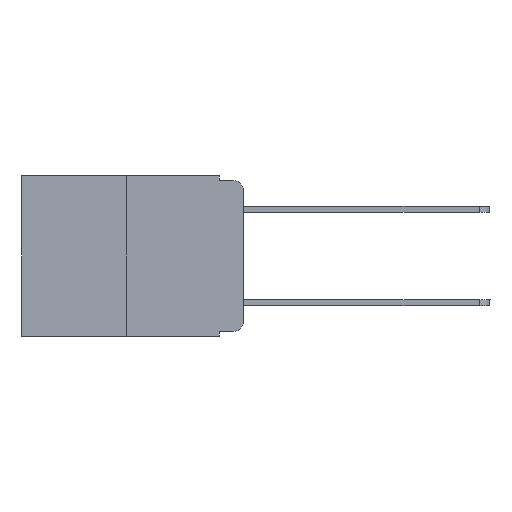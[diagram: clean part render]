
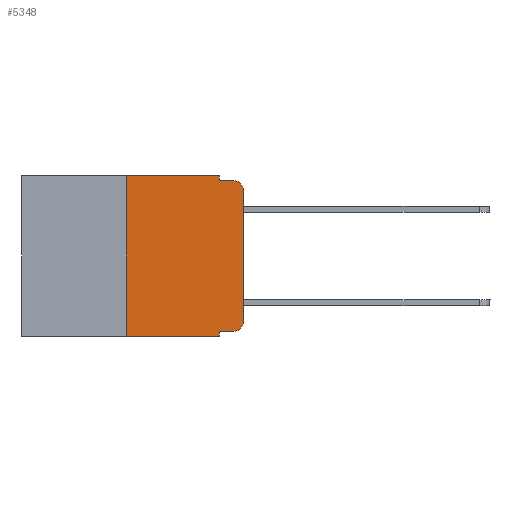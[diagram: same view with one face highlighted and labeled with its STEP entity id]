
A CAD part, left-side view. The second image highlights one B-rep face of the part: STEP entity #5348.
In plain terms, the highlighted planar face has unit normal (-1, 0, 0).
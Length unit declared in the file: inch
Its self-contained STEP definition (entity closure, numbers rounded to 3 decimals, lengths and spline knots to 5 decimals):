
#55 = VERTEX_POINT ( 'NONE', #11391 ) ;
#371 = DIRECTION ( 'NONE',  ( 0., -1., 0. ) ) ;
#463 = CARTESIAN_POINT ( 'NONE',  ( 0., 0.051, -0.01 ) ) ;
#691 = ORIENTED_EDGE ( 'NONE', *, *, #2611, .T. ) ;
#784 = VERTEX_POINT ( 'NONE', #4532 ) ;
#833 = EDGE_CURVE ( 'NONE', #9149, #11149, #3666, .T. ) ;
#1502 = CARTESIAN_POINT ( 'NONE',  ( 0., 0.473, -0.343 ) ) ;
#1610 = PLANE ( 'NONE',  #10020 ) ;
#1618 = CIRCLE ( 'NONE', #2426, 0.02 ) ;
#1732 = CARTESIAN_POINT ( 'NONE',  ( 0., 0., -0.313 ) ) ;
#1734 = DIRECTION ( 'NONE',  ( 0., 0., -1. ) ) ;
#2113 = VERTEX_POINT ( 'NONE', #3865 ) ;
#2253 = CARTESIAN_POINT ( 'NONE',  ( 0., 0.02, -0.333 ) ) ;
#2263 = EDGE_CURVE ( 'NONE', #55, #4100, #9160, .T. ) ;
#2370 = EDGE_CURVE ( 'NONE', #4100, #2113, #8452, .T. ) ;
#2426 = AXIS2_PLACEMENT_3D ( 'NONE', #6233, #11072, #10135 ) ;
#2611 = EDGE_CURVE ( 'NONE', #5269, #11379, #9604, .T. ) ;
#2740 = EDGE_CURVE ( 'NONE', #9149, #55, #5394, .T. ) ;
#3147 = CARTESIAN_POINT ( 'NONE',  ( 0., 0.051, 0. ) ) ;
#3274 = CARTESIAN_POINT ( 'NONE',  ( 0., 0.473, 0. ) ) ;
#3375 = CARTESIAN_POINT ( 'NONE',  ( 0., 0., 0. ) ) ;
#3553 = ORIENTED_EDGE ( 'NONE', *, *, #2263, .F. ) ;
#3666 = LINE ( 'NONE', #1502, #6670 ) ;
#3865 = CARTESIAN_POINT ( 'NONE',  ( 0., 0.051, -0.01 ) ) ;
#3949 = ORIENTED_EDGE ( 'NONE', *, *, #2370, .F. ) ;
#3954 = VECTOR ( 'NONE', #371, 39.37008 ) ;
#4019 = DIRECTION ( 'NONE',  ( 0., -1., 0. ) ) ;
#4100 = VERTEX_POINT ( 'NONE', #8369 ) ;
#4251 = DIRECTION ( 'NONE',  ( 0., 0., -1. ) ) ;
#4281 = EDGE_CURVE ( 'NONE', #784, #5269, #8822, .T. ) ;
#4304 = VERTEX_POINT ( 'NONE', #4315 ) ;
#4315 = CARTESIAN_POINT ( 'NONE',  ( 0., 0.02, -0.01 ) ) ;
#4472 = DIRECTION ( 'NONE',  ( 0., -1., 0. ) ) ;
#4532 = CARTESIAN_POINT ( 'NONE',  ( 0., 0.051, -0.333 ) ) ;
#4539 = VECTOR ( 'NONE', #8226, 39.37008 ) ;
#4575 = VECTOR ( 'NONE', #9256, 39.37008 ) ;
#4595 = VECTOR ( 'NONE', #9797, 39.37008 ) ;
#4794 = VECTOR ( 'NONE', #4019, 39.37008 ) ;
#4925 = CARTESIAN_POINT ( 'NONE',  ( 0., 0.051, -0.343 ) ) ;
#5269 = VERTEX_POINT ( 'NONE', #2253 ) ;
#5348 = ADVANCED_FACE ( 'NONE', ( #6421 ), #1610, .F. ) ;
#5394 = LINE ( 'NONE', #9311, #4539 ) ;
#5399 = LINE ( 'NONE', #3375, #4575 ) ;
#5636 = VECTOR ( 'NONE', #11295, 39.37008 ) ;
#6051 = EDGE_CURVE ( 'NONE', #11379, #7985, #5399, .T. ) ;
#6233 = CARTESIAN_POINT ( 'NONE',  ( 0., 0.02, -0.03 ) ) ;
#6367 = ORIENTED_EDGE ( 'NONE', *, *, #4281, .T. ) ;
#6421 = FACE_OUTER_BOUND ( 'NONE', #12155, .T. ) ;
#6670 = VECTOR ( 'NONE', #4472, 39.37008 ) ;
#6809 = CARTESIAN_POINT ( 'NONE',  ( 0., 0.02, -0.313 ) ) ;
#6917 = CARTESIAN_POINT ( 'NONE',  ( 0., 0.25, -0.343 ) ) ;
#6931 = EDGE_CURVE ( 'NONE', #784, #11149, #11745, .T. ) ;
#7358 = AXIS2_PLACEMENT_3D ( 'NONE', #6809, #11062, #4251 ) ;
#7933 = EDGE_CURVE ( 'NONE', #2113, #4304, #9127, .T. ) ;
#7985 = VERTEX_POINT ( 'NONE', #11174 ) ;
#8226 = DIRECTION ( 'NONE',  ( 0., 0., 1. ) ) ;
#8311 = CARTESIAN_POINT ( 'NONE',  ( 0., 0.473, 0. ) ) ;
#8369 = CARTESIAN_POINT ( 'NONE',  ( 0., 0.051, 0. ) ) ;
#8452 = LINE ( 'NONE', #10273, #10597 ) ;
#8738 = ORIENTED_EDGE ( 'NONE', *, *, #7933, .F. ) ;
#8822 = LINE ( 'NONE', #10643, #4794 ) ;
#9127 = LINE ( 'NONE', #463, #5636 ) ;
#9149 = VERTEX_POINT ( 'NONE', #6917 ) ;
#9160 = LINE ( 'NONE', #3274, #3954 ) ;
#9256 = DIRECTION ( 'NONE',  ( 0., 0., 1. ) ) ;
#9311 = CARTESIAN_POINT ( 'NONE',  ( 0., 0.25, 0. ) ) ;
#9314 = EDGE_CURVE ( 'NONE', #7985, #4304, #1618, .T. ) ;
#9579 = ORIENTED_EDGE ( 'NONE', *, *, #6051, .T. ) ;
#9604 = CIRCLE ( 'NONE', #7358, 0.02 ) ;
#9690 = ORIENTED_EDGE ( 'NONE', *, *, #9314, .T. ) ;
#9763 = ORIENTED_EDGE ( 'NONE', *, *, #6931, .F. ) ;
#9797 = DIRECTION ( 'NONE',  ( 0., 0., -1. ) ) ;
#10020 = AXIS2_PLACEMENT_3D ( 'NONE', #8311, #10389, #1734 ) ;
#10135 = DIRECTION ( 'NONE',  ( 0., 0., -1. ) ) ;
#10273 = CARTESIAN_POINT ( 'NONE',  ( 0., 0.051, 0. ) ) ;
#10389 = DIRECTION ( 'NONE',  ( 1., 0., 0. ) ) ;
#10597 = VECTOR ( 'NONE', #12282, 39.37008 ) ;
#10643 = CARTESIAN_POINT ( 'NONE',  ( 0., 0.051, -0.333 ) ) ;
#11062 = DIRECTION ( 'NONE',  ( -1., 0., 0. ) ) ;
#11072 = DIRECTION ( 'NONE',  ( -1., 0., 0. ) ) ;
#11149 = VERTEX_POINT ( 'NONE', #4925 ) ;
#11174 = CARTESIAN_POINT ( 'NONE',  ( 0., 0., -0.03 ) ) ;
#11295 = DIRECTION ( 'NONE',  ( 0., -1., 0. ) ) ;
#11379 = VERTEX_POINT ( 'NONE', #1732 ) ;
#11391 = CARTESIAN_POINT ( 'NONE',  ( 0., 0.25, 0. ) ) ;
#11561 = ORIENTED_EDGE ( 'NONE', *, *, #833, .T. ) ;
#11694 = ORIENTED_EDGE ( 'NONE', *, *, #2740, .F. ) ;
#11745 = LINE ( 'NONE', #3147, #4595 ) ;
#12155 = EDGE_LOOP ( 'NONE', ( #9579, #9690, #8738, #3949, #3553, #11694, #11561, #9763, #6367, #691 ) ) ;
#12282 = DIRECTION ( 'NONE',  ( 0., 0., -1. ) ) ;
